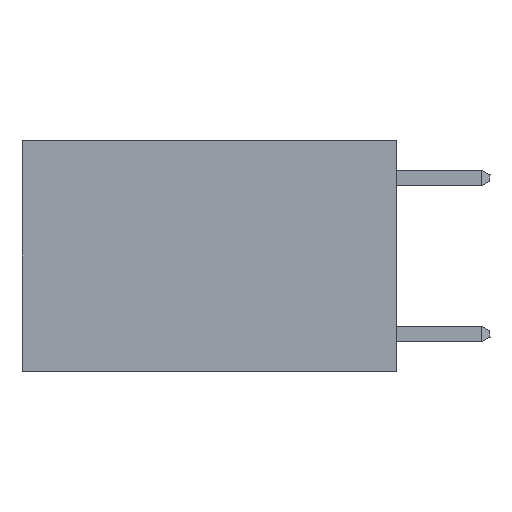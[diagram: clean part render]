
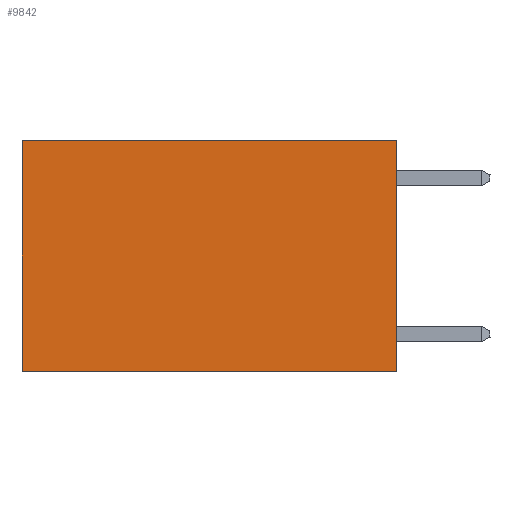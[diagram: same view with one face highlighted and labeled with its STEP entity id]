
A CAD part, left-side view. The second image highlights one B-rep face of the part: STEP entity #9842.
In plain terms, the highlighted planar face has unit normal (-1, 0, 0).
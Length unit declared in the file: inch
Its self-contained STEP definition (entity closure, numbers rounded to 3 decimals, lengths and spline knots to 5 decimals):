
#178 = EDGE_CURVE ( 'NONE', #9078, #2568, #4036, .T. ) ;
#211 = EDGE_CURVE ( 'NONE', #3958, #9078, #2799, .T. ) ;
#394 = CARTESIAN_POINT ( 'NONE',  ( 0.2625, 0., 0. ) ) ;
#560 = DIRECTION ( 'NONE',  ( 0., 0., -1. ) ) ;
#1093 = CARTESIAN_POINT ( 'NONE',  ( 0.2625, 0., 0. ) ) ;
#1259 = CARTESIAN_POINT ( 'NONE',  ( 0.2625, 0.6, 0. ) ) ;
#1447 = EDGE_LOOP ( 'NONE', ( #4830, #3084, #14729, #7677 ) ) ;
#1759 = VECTOR ( 'NONE', #14256, 39.37008 ) ;
#1911 = CARTESIAN_POINT ( 'NONE',  ( 0.2625, 0., -0.37 ) ) ;
#2460 = LINE ( 'NONE', #8088, #1759 ) ;
#2568 = VERTEX_POINT ( 'NONE', #3042 ) ;
#2799 = LINE ( 'NONE', #394, #8781 ) ;
#3042 = CARTESIAN_POINT ( 'NONE',  ( 0.2625, 0.6, -0.37 ) ) ;
#3084 = ORIENTED_EDGE ( 'NONE', *, *, #11349, .F. ) ;
#3831 = DIRECTION ( 'NONE',  ( 1., 0., 0. ) ) ;
#3958 = VERTEX_POINT ( 'NONE', #12379 ) ;
#4036 = LINE ( 'NONE', #9898, #7534 ) ;
#4178 = VECTOR ( 'NONE', #13701, 39.37008 ) ;
#4752 = PLANE ( 'NONE',  #8590 ) ;
#4830 = ORIENTED_EDGE ( 'NONE', *, *, #178, .T. ) ;
#6057 = CARTESIAN_POINT ( 'NONE',  ( 0.2625, 0., 0. ) ) ;
#7534 = VECTOR ( 'NONE', #560, 39.37008 ) ;
#7677 = ORIENTED_EDGE ( 'NONE', *, *, #211, .T. ) ;
#8088 = CARTESIAN_POINT ( 'NONE',  ( 0.2625, 0., -0.37 ) ) ;
#8590 = AXIS2_PLACEMENT_3D ( 'NONE', #6057, #3831, #13180 ) ;
#8781 = VECTOR ( 'NONE', #12136, 39.37008 ) ;
#9015 = LINE ( 'NONE', #1093, #4178 ) ;
#9078 = VERTEX_POINT ( 'NONE', #1259 ) ;
#9842 = ADVANCED_FACE ( 'NONE', ( #12017 ), #4752, .F. ) ;
#9898 = CARTESIAN_POINT ( 'NONE',  ( 0.2625, 0.6, 0. ) ) ;
#11166 = VERTEX_POINT ( 'NONE', #1911 ) ;
#11349 = EDGE_CURVE ( 'NONE', #11166, #2568, #2460, .T. ) ;
#12017 = FACE_OUTER_BOUND ( 'NONE', #1447, .T. ) ;
#12136 = DIRECTION ( 'NONE',  ( 0., 1., 0. ) ) ;
#12379 = CARTESIAN_POINT ( 'NONE',  ( 0.2625, 0., 0. ) ) ;
#13180 = DIRECTION ( 'NONE',  ( 0., 0., -1. ) ) ;
#13493 = EDGE_CURVE ( 'NONE', #3958, #11166, #9015, .T. ) ;
#13701 = DIRECTION ( 'NONE',  ( 0., 0., -1. ) ) ;
#14256 = DIRECTION ( 'NONE',  ( 0., 1., 0. ) ) ;
#14729 = ORIENTED_EDGE ( 'NONE', *, *, #13493, .F. ) ;
